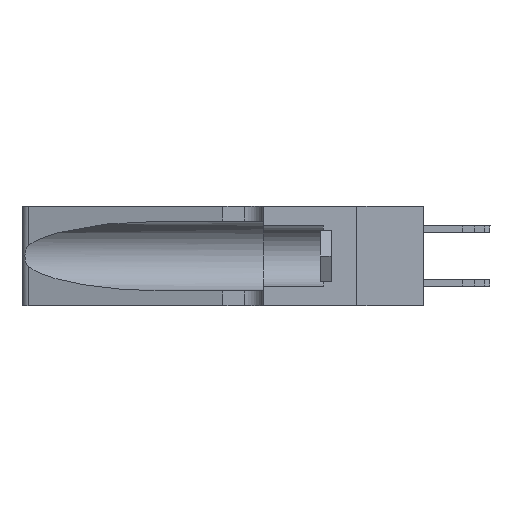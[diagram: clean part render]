
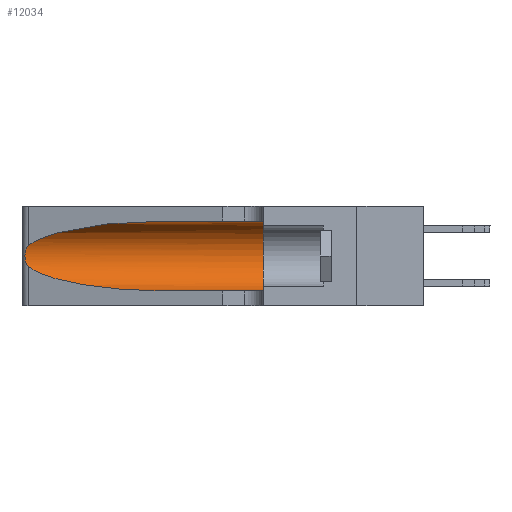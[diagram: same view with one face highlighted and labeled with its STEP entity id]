
A CAD part, left-side view. The second image highlights one B-rep face of the part: STEP entity #12034.
In plain terms, the highlighted cylindrical face has radius 3.308 mm (diameter 6.617 mm), a partial arc.
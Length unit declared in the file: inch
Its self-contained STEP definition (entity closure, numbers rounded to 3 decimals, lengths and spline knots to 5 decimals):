
#26 = VECTOR ( 'NONE', #214, 39.37008 ) ;
#214 = DIRECTION ( 'NONE',  ( 0., -1., 0. ) ) ;
#309 = CARTESIAN_POINT ( 'NONE',  ( 0.26075, 1.23896, 0.178 ) ) ;
#1013 = DIRECTION ( 'NONE',  ( 0., 1., 0. ) ) ;
#1658 = CARTESIAN_POINT ( 'NONE',  ( 0.25487, 1.22718, 0.14631 ) ) ;
#1761 = CARTESIAN_POINT ( 'NONE',  ( 0.2373, 1.15595, 0.08982 ) ) ;
#1913 = CARTESIAN_POINT ( 'NONE',  ( 0.25854, 1.2359, 0.20912 ) ) ;
#1953 = CIRCLE ( 'NONE', #2558, 0.13025 ) ;
#2558 = AXIS2_PLACEMENT_3D ( 'NONE', #6841, #1013, #20237 ) ;
#3541 = EDGE_CURVE ( 'NONE', #23890, #16879, #10828, .T. ) ;
#3872 = CARTESIAN_POINT ( 'NONE',  ( 0.26018, 1.23835, 0.19895 ) ) ;
#3911 = CARTESIAN_POINT ( 'NONE',  ( 0.1305, 0.72297, 0.31525 ) ) ;
#4443 =( BOUNDED_CURVE ( )  B_SPLINE_CURVE ( 3, ( #5742, #1761, #9722, #23434 ),
 .UNSPECIFIED., .F., .T. ) 
 B_SPLINE_CURVE_WITH_KNOTS ( ( 4, 4 ),
 ( 3.44316, 4.71239 ),
 .UNSPECIFIED. ) 
 CURVE ( )  GEOMETRIC_REPRESENTATION_ITEM ( )  RATIONAL_B_SPLINE_CURVE ( ( 1., 0.87, 0.87, 1. ) ) 
 REPRESENTATION_ITEM ( '' )  );
#4832 = AXIS2_PLACEMENT_3D ( 'NONE', #8621, #22272, #10610 ) ;
#5742 = CARTESIAN_POINT ( 'NONE',  ( 0.25487, 1.22718, 0.14631 ) ) ;
#6227 = CARTESIAN_POINT ( 'NONE',  ( 0.25856, 1.23593, 0.16098 ) ) ;
#6841 = CARTESIAN_POINT ( 'NONE',  ( 0.1305, 0.35, 0.185 ) ) ;
#7025 = EDGE_CURVE ( 'NONE', #8705, #12636, #7116, .T. ) ;
#7116 = B_SPLINE_CURVE_WITH_KNOTS ( 'NONE', 3,
 ( #18559, #18644, #25317, #25280, #1913, #3872, #23746, #309, #13804, #6227, #17942, #19811, #21875, #7880 ),
 .UNSPECIFIED., .F., .F.,
 ( 4, 2, 2, 2, 2, 2, 4 ),
 ( 0., 0.00027, 0.00053, 0.00107, 0.0016, 0.00187, 0.00214 ),
 .UNSPECIFIED. ) ;
#7412 = CARTESIAN_POINT ( 'NONE',  ( 0.1305, 1.61858, 0.05475 ) ) ;
#7714 = CYLINDRICAL_SURFACE ( 'NONE', #4832, 0.13025 ) ;
#7780 = CARTESIAN_POINT ( 'NONE',  ( 0.1305, 1.61858, 0.31525 ) ) ;
#7880 = CARTESIAN_POINT ( 'NONE',  ( 0.25487, 1.22718, 0.14631 ) ) ;
#8311 = CARTESIAN_POINT ( 'NONE',  ( 0.1305, 0.72297, 0.31525 ) ) ;
#8621 = CARTESIAN_POINT ( 'NONE',  ( 0.1305, 1.61858, 0.185 ) ) ;
#8705 = VERTEX_POINT ( 'NONE', #17163 ) ;
#8845 = ORIENTED_EDGE ( 'NONE', *, *, #14764, .F. ) ;
#9375 = ORIENTED_EDGE ( 'NONE', *, *, #7025, .T. ) ;
#9500 = ORIENTED_EDGE ( 'NONE', *, *, #13907, .F. ) ;
#9722 = CARTESIAN_POINT ( 'NONE',  ( 0.18966, 0.96281, 0.05475 ) ) ;
#9950 = VECTOR ( 'NONE', #19277, 39.37008 ) ;
#10246 = VERTEX_POINT ( 'NONE', #8311 ) ;
#10465 = LINE ( 'NONE', #7780, #26 ) ;
#10610 = DIRECTION ( 'NONE',  ( 0., 0., -1. ) ) ;
#10828 = LINE ( 'NONE', #7412, #9950 ) ;
#11460 = CARTESIAN_POINT ( 'NONE',  ( 0.25487, 1.22718, 0.22369 ) ) ;
#12034 = ADVANCED_FACE ( 'NONE', ( #15680 ), #7714, .F. ) ;
#12432 =( BOUNDED_CURVE ( )  B_SPLINE_CURVE ( 3, ( #3911, #13592, #14722, #11460 ),
 .UNSPECIFIED., .F., .T. ) 
 B_SPLINE_CURVE_WITH_KNOTS ( ( 4, 4 ),
 ( 1.5708, 2.84003 ),
 .UNSPECIFIED. ) 
 CURVE ( )  GEOMETRIC_REPRESENTATION_ITEM ( )  RATIONAL_B_SPLINE_CURVE ( ( 1., 0.87, 0.87, 1. ) ) 
 REPRESENTATION_ITEM ( '' )  );
#12636 = VERTEX_POINT ( 'NONE', #1658 ) ;
#13592 = CARTESIAN_POINT ( 'NONE',  ( 0.18966, 0.96281, 0.31525 ) ) ;
#13804 = CARTESIAN_POINT ( 'NONE',  ( 0.26017, 1.23833, 0.17102 ) ) ;
#13907 = EDGE_CURVE ( 'NONE', #23306, #16879, #1953, .T. ) ;
#14616 = CARTESIAN_POINT ( 'NONE',  ( 0.1305, 0.72297, 0.05475 ) ) ;
#14629 = ORIENTED_EDGE ( 'NONE', *, *, #15000, .T. ) ;
#14722 = CARTESIAN_POINT ( 'NONE',  ( 0.2373, 1.15595, 0.28018 ) ) ;
#14764 = EDGE_CURVE ( 'NONE', #10246, #23306, #10465, .T. ) ;
#15000 = EDGE_CURVE ( 'NONE', #10246, #8705, #12432, .T. ) ;
#15680 = FACE_OUTER_BOUND ( 'NONE', #19507, .T. ) ;
#16559 = CARTESIAN_POINT ( 'NONE',  ( 0.1305, 0.35, 0.31525 ) ) ;
#16879 = VERTEX_POINT ( 'NONE', #22673 ) ;
#17163 = CARTESIAN_POINT ( 'NONE',  ( 0.25487, 1.22718, 0.22369 ) ) ;
#17942 = CARTESIAN_POINT ( 'NONE',  ( 0.25789, 1.23486, 0.15765 ) ) ;
#18433 = EDGE_CURVE ( 'NONE', #12636, #23890, #4443, .T. ) ;
#18559 = CARTESIAN_POINT ( 'NONE',  ( 0.25487, 1.22718, 0.22369 ) ) ;
#18644 = CARTESIAN_POINT ( 'NONE',  ( 0.25555, 1.22994, 0.2215 ) ) ;
#19251 = ORIENTED_EDGE ( 'NONE', *, *, #3541, .T. ) ;
#19277 = DIRECTION ( 'NONE',  ( 0., -1., 0. ) ) ;
#19507 = EDGE_LOOP ( 'NONE', ( #14629, #9375, #22756, #19251, #9500, #8845 ) ) ;
#19811 = CARTESIAN_POINT ( 'NONE',  ( 0.25639, 1.23186, 0.15144 ) ) ;
#20237 = DIRECTION ( 'NONE',  ( 0., 0., 1. ) ) ;
#21875 = CARTESIAN_POINT ( 'NONE',  ( 0.25555, 1.22993, 0.14849 ) ) ;
#22272 = DIRECTION ( 'NONE',  ( 0., -1., 0. ) ) ;
#22673 = CARTESIAN_POINT ( 'NONE',  ( 0.1305, 0.35, 0.05475 ) ) ;
#22756 = ORIENTED_EDGE ( 'NONE', *, *, #18433, .T. ) ;
#23306 = VERTEX_POINT ( 'NONE', #16559 ) ;
#23434 = CARTESIAN_POINT ( 'NONE',  ( 0.1305, 0.72297, 0.05475 ) ) ;
#23746 = CARTESIAN_POINT ( 'NONE',  ( 0.26075, 1.23896, 0.19203 ) ) ;
#23890 = VERTEX_POINT ( 'NONE', #14616 ) ;
#25280 = CARTESIAN_POINT ( 'NONE',  ( 0.25787, 1.23484, 0.2124 ) ) ;
#25317 = CARTESIAN_POINT ( 'NONE',  ( 0.25639, 1.23184, 0.21858 ) ) ;
